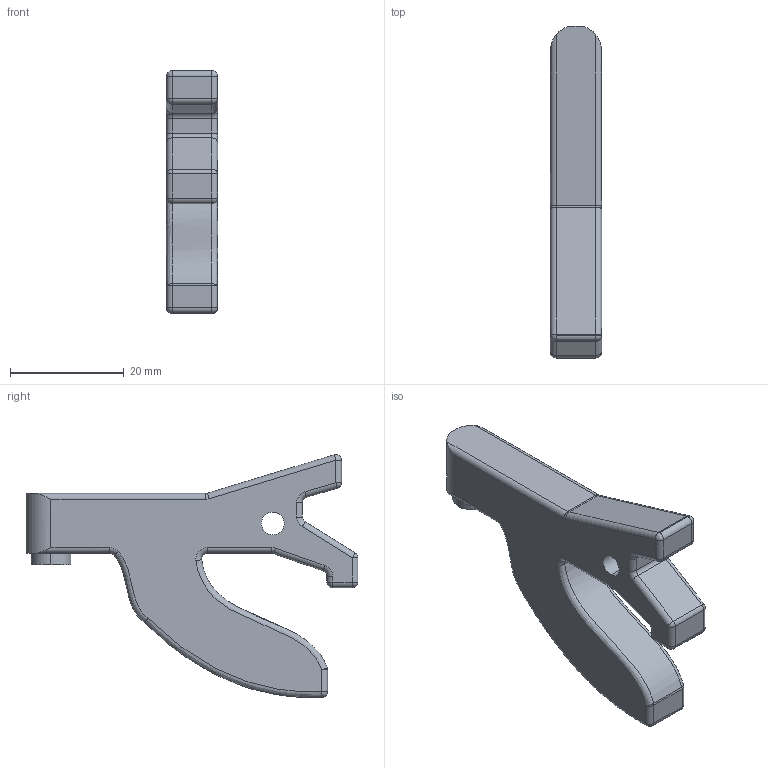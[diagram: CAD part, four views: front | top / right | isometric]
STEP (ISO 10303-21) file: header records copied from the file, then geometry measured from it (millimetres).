
FILE_DESCRIPTION (( 'STEP AP203' ), '1' );
FILE_NAME ('final_hammer.STEP', '2013-07-12T02:44:59', ( '' ), ( '' ), 'SwSTEP 2.0', 'SolidWorks 2012', '' );
FILE_SCHEMA (( 'CONFIG_CONTROL_DESIGN' ));
Length unit declared in the file: millimetre
Products named in the file (1): final_hammer
Bounding box: 9 x 58.36 x 42.73 mm (x, y, z)
Volume: 10110 mm3; surface area: 4261.3 mm2
Topology: 1 solids, 1 shells, 105 faces, 245 edges, 128 vertices
Faces by surface type: cylinder 48, plane 19, sphere 15, torus 14, bspline 9
Entity records: 3705 total; most frequent: CARTESIAN_POINT 1322, DIRECTION 522, ORIENTED_EDGE 462, EDGE_CURVE 231, AXIS2_PLACEMENT_3D 212, VERTEX_POINT 128, CIRCLE 115, EDGE_LOOP 107
